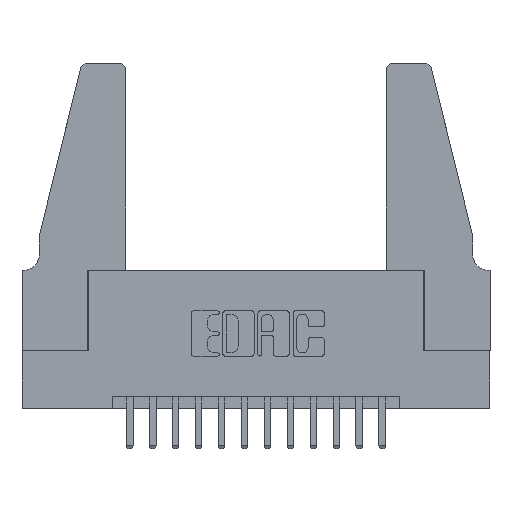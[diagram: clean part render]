
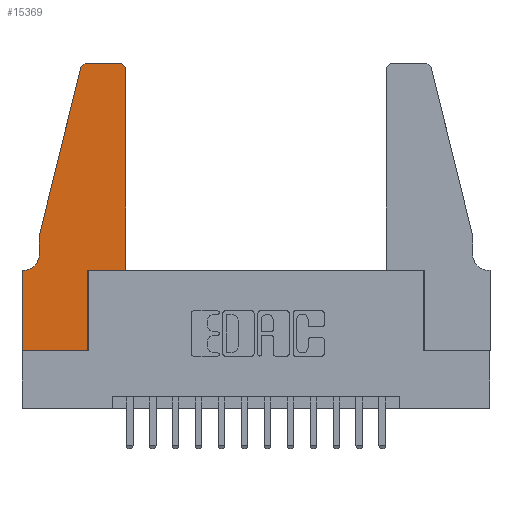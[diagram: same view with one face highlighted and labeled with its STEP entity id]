
A CAD part, top view. The second image highlights one B-rep face of the part: STEP entity #15369.
In plain terms, the highlighted planar face has unit normal (0, 0, 1).
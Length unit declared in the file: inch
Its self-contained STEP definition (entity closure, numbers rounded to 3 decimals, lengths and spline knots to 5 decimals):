
#61 = EDGE_CURVE ( 'NONE', #8534, #324, #4386, .T. ) ;
#170 = DIRECTION ( 'NONE',  ( 0., 0., -1. ) ) ;
#209 = DIRECTION ( 'NONE',  ( -1., 0., 0. ) ) ;
#324 = VERTEX_POINT ( 'NONE', #10332 ) ;
#408 = CARTESIAN_POINT ( 'NONE',  ( 0.0055, 0.42, 0.37 ) ) ;
#1015 = VERTEX_POINT ( 'NONE', #11909 ) ;
#1049 = EDGE_CURVE ( 'NONE', #1800, #6766, #3358, .T. ) ;
#1210 = DIRECTION ( 'NONE',  ( 0., 1., 0. ) ) ;
#1548 = CIRCLE ( 'NONE', #3839, 0.03 ) ;
#1660 = CARTESIAN_POINT ( 'NONE',  ( 0.4505, 1.22, 0.37 ) ) ;
#1663 = EDGE_CURVE ( 'NONE', #1015, #9824, #7571, .T. ) ;
#1782 = DIRECTION ( 'NONE',  ( 0., 0., 1. ) ) ;
#1800 = VERTEX_POINT ( 'NONE', #13978 ) ;
#2131 = VERTEX_POINT ( 'NONE', #11090 ) ;
#2310 = EDGE_CURVE ( 'NONE', #8596, #1015, #11542, .T. ) ;
#2480 = CARTESIAN_POINT ( 'NONE',  ( 0.0755, 0.5, 0.37 ) ) ;
#2550 = ORIENTED_EDGE ( 'NONE', *, *, #12026, .T. ) ;
#2596 = CIRCLE ( 'NONE', #11677, 0.03 ) ;
#2703 = CARTESIAN_POINT ( 'NONE',  ( 0.4505, 0.35, 0.37 ) ) ;
#3008 = CARTESIAN_POINT ( 'NONE',  ( 0.25487, 1.22718, 0.37 ) ) ;
#3025 = AXIS2_PLACEMENT_3D ( 'NONE', #408, #170, #209 ) ;
#3035 = LINE ( 'NONE', #10813, #15186 ) ;
#3214 = LINE ( 'NONE', #12414, #12565 ) ;
#3358 = LINE ( 'NONE', #2703, #9462 ) ;
#3512 = DIRECTION ( 'NONE',  ( 0., 1., 0. ) ) ;
#3839 = AXIS2_PLACEMENT_3D ( 'NONE', #9109, #1782, #10305 ) ;
#3895 = DIRECTION ( 'NONE',  ( 1., 0., 0. ) ) ;
#4303 = CARTESIAN_POINT ( 'NONE',  ( 0., 0.35, 0.37 ) ) ;
#4386 = LINE ( 'NONE', #13385, #7256 ) ;
#4477 = CARTESIAN_POINT ( 'NONE',  ( 0.4505, 0.35, 0.37 ) ) ;
#4519 = ORIENTED_EDGE ( 'NONE', *, *, #1049, .T. ) ;
#4886 = ORIENTED_EDGE ( 'NONE', *, *, #15342, .T. ) ;
#5380 = LINE ( 'NONE', #9108, #14247 ) ;
#5576 = DIRECTION ( 'NONE',  ( 1., 0., 0. ) ) ;
#5665 = DIRECTION ( 'NONE',  ( 0., 0., 1. ) ) ;
#5856 = LINE ( 'NONE', #6105, #8697 ) ;
#5858 = VERTEX_POINT ( 'NONE', #6217 ) ;
#6105 = CARTESIAN_POINT ( 'NONE',  ( 0.4505, 0.35, 0.37 ) ) ;
#6111 = VERTEX_POINT ( 'NONE', #3008 ) ;
#6215 = ORIENTED_EDGE ( 'NONE', *, *, #7421, .T. ) ;
#6217 = CARTESIAN_POINT ( 'NONE',  ( 0.284, 1.25, 0.37 ) ) ;
#6459 = ORIENTED_EDGE ( 'NONE', *, *, #10439, .T. ) ;
#6591 = ORIENTED_EDGE ( 'NONE', *, *, #8391, .T. ) ;
#6766 = VERTEX_POINT ( 'NONE', #4477 ) ;
#7256 = VECTOR ( 'NONE', #15272, 39.37008 ) ;
#7281 = VERTEX_POINT ( 'NONE', #1660 ) ;
#7421 = EDGE_CURVE ( 'NONE', #5858, #6111, #2596, .T. ) ;
#7467 = VECTOR ( 'NONE', #11874, 39.37008 ) ;
#7571 = CIRCLE ( 'NONE', #3025, 0.07 ) ;
#7828 = FACE_OUTER_BOUND ( 'NONE', #10151, .T. ) ;
#7838 = LINE ( 'NONE', #10653, #7467 ) ;
#7930 = VECTOR ( 'NONE', #13442, 39.37008 ) ;
#8339 = VECTOR ( 'NONE', #10983, 39.37008 ) ;
#8343 = EDGE_CURVE ( 'NONE', #6766, #7281, #5856, .T. ) ;
#8391 = EDGE_CURVE ( 'NONE', #6111, #8596, #11900, .T. ) ;
#8534 = VERTEX_POINT ( 'NONE', #11536 ) ;
#8543 = ORIENTED_EDGE ( 'NONE', *, *, #61, .T. ) ;
#8596 = VERTEX_POINT ( 'NONE', #12861 ) ;
#8697 = VECTOR ( 'NONE', #1210, 39.37008 ) ;
#9052 = ORIENTED_EDGE ( 'NONE', *, *, #14380, .T. ) ;
#9109 = CARTESIAN_POINT ( 'NONE',  ( 0.4205, 1.22, 0.37 ) ) ;
#9108 = CARTESIAN_POINT ( 'NONE',  ( 0.0755, 0.35, 0.37 ) ) ;
#9126 = CARTESIAN_POINT ( 'NONE',  ( 0.0055, 0.35, 0.37 ) ) ;
#9462 = VECTOR ( 'NONE', #11844, 39.37008 ) ;
#9824 = VERTEX_POINT ( 'NONE', #9126 ) ;
#10151 = EDGE_LOOP ( 'NONE', ( #9052, #6215, #6591, #13016, #13785, #4886, #8543, #12126, #2550, #4519, #15057, #6459 ) ) ;
#10305 = DIRECTION ( 'NONE',  ( 1., 0., 0. ) ) ;
#10332 = CARTESIAN_POINT ( 'NONE',  ( 0., 0., 0.37 ) ) ;
#10439 = EDGE_CURVE ( 'NONE', #7281, #11346, #1548, .T. ) ;
#10653 = CARTESIAN_POINT ( 'NONE',  ( 0.2605, 1.25, 0.37 ) ) ;
#10813 = CARTESIAN_POINT ( 'NONE',  ( 0.2865, 0.35, 0.37 ) ) ;
#10983 = DIRECTION ( 'NONE',  ( 0., -1., 0. ) ) ;
#11090 = CARTESIAN_POINT ( 'NONE',  ( 0.2865, 0., 0.37 ) ) ;
#11346 = VERTEX_POINT ( 'NONE', #12151 ) ;
#11485 = DIRECTION ( 'NONE',  ( -1., 0., 0. ) ) ;
#11528 = CARTESIAN_POINT ( 'NONE',  ( 0.0755, 0.5, 0.37 ) ) ;
#11536 = CARTESIAN_POINT ( 'NONE',  ( 0., 0.35, 0.37 ) ) ;
#11542 = LINE ( 'NONE', #11528, #8339 ) ;
#11588 = PLANE ( 'NONE',  #13959 ) ;
#11677 = AXIS2_PLACEMENT_3D ( 'NONE', #12890, #5665, #14103 ) ;
#11844 = DIRECTION ( 'NONE',  ( 1., 0., 0. ) ) ;
#11874 = DIRECTION ( 'NONE',  ( -1., 0., 0. ) ) ;
#11900 = LINE ( 'NONE', #2480, #7930 ) ;
#11909 = CARTESIAN_POINT ( 'NONE',  ( 0.0755, 0.42, 0.37 ) ) ;
#12026 = EDGE_CURVE ( 'NONE', #2131, #1800, #3035, .T. ) ;
#12126 = ORIENTED_EDGE ( 'NONE', *, *, #14670, .T. ) ;
#12151 = CARTESIAN_POINT ( 'NONE',  ( 0.4205, 1.25, 0.37 ) ) ;
#12414 = CARTESIAN_POINT ( 'NONE',  ( 0., 0., 0.37 ) ) ;
#12565 = VECTOR ( 'NONE', #3895, 39.37008 ) ;
#12808 = DIRECTION ( 'NONE',  ( 0., 0., 1. ) ) ;
#12861 = CARTESIAN_POINT ( 'NONE',  ( 0.0755, 0.5, 0.37 ) ) ;
#12890 = CARTESIAN_POINT ( 'NONE',  ( 0.284, 1.22, 0.37 ) ) ;
#13016 = ORIENTED_EDGE ( 'NONE', *, *, #2310, .T. ) ;
#13385 = CARTESIAN_POINT ( 'NONE',  ( 0., 0., 0.37 ) ) ;
#13442 = DIRECTION ( 'NONE',  ( -0.239, -0.971, 0. ) ) ;
#13785 = ORIENTED_EDGE ( 'NONE', *, *, #1663, .T. ) ;
#13959 = AXIS2_PLACEMENT_3D ( 'NONE', #4303, #12808, #5576 ) ;
#13978 = CARTESIAN_POINT ( 'NONE',  ( 0.2865, 0.35, 0.37 ) ) ;
#14103 = DIRECTION ( 'NONE',  ( 1., 0., 0. ) ) ;
#14247 = VECTOR ( 'NONE', #11485, 39.37008 ) ;
#14380 = EDGE_CURVE ( 'NONE', #11346, #5858, #7838, .T. ) ;
#14670 = EDGE_CURVE ( 'NONE', #324, #2131, #3214, .T. ) ;
#15057 = ORIENTED_EDGE ( 'NONE', *, *, #8343, .T. ) ;
#15186 = VECTOR ( 'NONE', #3512, 39.37008 ) ;
#15272 = DIRECTION ( 'NONE',  ( 0., -1., 0. ) ) ;
#15342 = EDGE_CURVE ( 'NONE', #9824, #8534, #5380, .T. ) ;
#15369 = ADVANCED_FACE ( 'NONE', ( #7828 ), #11588, .T. ) ;
